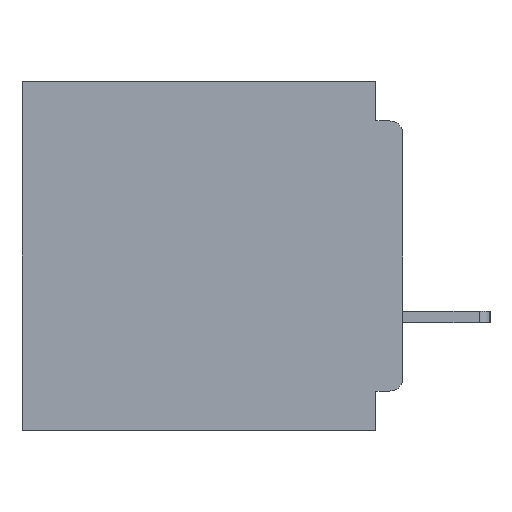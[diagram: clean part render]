
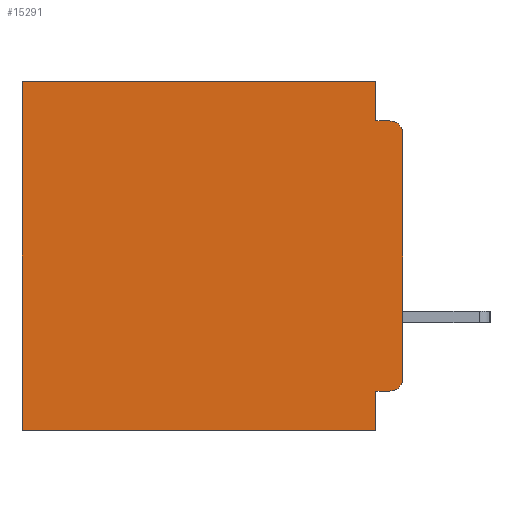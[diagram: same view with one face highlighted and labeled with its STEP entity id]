
A CAD part, left-side view. The second image highlights one B-rep face of the part: STEP entity #15291.
In plain terms, the highlighted planar face has unit normal (-1, 0, 0).
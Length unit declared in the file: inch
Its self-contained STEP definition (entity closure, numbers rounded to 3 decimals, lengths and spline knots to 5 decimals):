
#118 = VERTEX_POINT ( 'NONE', #8648 ) ;
#592 = CARTESIAN_POINT ( 'NONE',  ( 0.3, 0.015, -0.34 ) ) ;
#712 = LINE ( 'NONE', #7384, #21413 ) ;
#1091 = DIRECTION ( 'NONE',  ( 0., -1., 0. ) ) ;
#1253 = EDGE_CURVE ( 'NONE', #20576, #32016, #34575, .T. ) ;
#2187 = EDGE_CURVE ( 'NONE', #118, #33348, #6329, .T. ) ;
#2341 = LINE ( 'NONE', #9358, #29979 ) ;
#2576 = ORIENTED_EDGE ( 'NONE', *, *, #2187, .F. ) ;
#2842 = ORIENTED_EDGE ( 'NONE', *, *, #1253, .F. ) ;
#3294 = ORIENTED_EDGE ( 'NONE', *, *, #25798, .T. ) ;
#3337 = ORIENTED_EDGE ( 'NONE', *, *, #29165, .F. ) ;
#3366 = DIRECTION ( 'NONE',  ( 0., 0., -1. ) ) ;
#4216 = CARTESIAN_POINT ( 'NONE',  ( 0.3, 0., -0.34 ) ) ;
#4332 = CARTESIAN_POINT ( 'NONE',  ( 0.3, 0., -0.4 ) ) ;
#4513 = CARTESIAN_POINT ( 'NONE',  ( 0.3, 0.437, -0.4 ) ) ;
#4587 = VERTEX_POINT ( 'NONE', #31724 ) ;
#4635 = CARTESIAN_POINT ( 'NONE',  ( 0.3, 0.031, -0.4 ) ) ;
#5099 = LINE ( 'NONE', #10769, #32546 ) ;
#5153 = ORIENTED_EDGE ( 'NONE', *, *, #20494, .F. ) ;
#5344 = CARTESIAN_POINT ( 'NONE',  ( 0.3, 0., -0.355 ) ) ;
#5604 = DIRECTION ( 'NONE',  ( -1., 0., 0. ) ) ;
#6329 = LINE ( 'NONE', #8721, #26789 ) ;
#6589 = LINE ( 'NONE', #4332, #33174 ) ;
#7053 = DIRECTION ( 'NONE',  ( 0., 1., 0. ) ) ;
#7383 = CARTESIAN_POINT ( 'NONE',  ( 0.3, 0., -0.4 ) ) ;
#7384 = CARTESIAN_POINT ( 'NONE',  ( 0.3, 0.031, 0. ) ) ;
#7402 = EDGE_CURVE ( 'NONE', #33550, #20576, #712, .T. ) ;
#8648 = CARTESIAN_POINT ( 'NONE',  ( 0.3, 0.031, -0.355 ) ) ;
#8721 = CARTESIAN_POINT ( 'NONE',  ( 0.3, 0.031, -0.4 ) ) ;
#9358 = CARTESIAN_POINT ( 'NONE',  ( 0.3, 0.437, -0.4 ) ) ;
#9608 = CIRCLE ( 'NONE', #10340, 0.015 ) ;
#9758 = VECTOR ( 'NONE', #10749, 39.37008 ) ;
#10077 = DIRECTION ( 'NONE',  ( 0., 0., -1. ) ) ;
#10340 = AXIS2_PLACEMENT_3D ( 'NONE', #21699, #5604, #24357 ) ;
#10695 = EDGE_CURVE ( 'NONE', #22828, #118, #16925, .T. ) ;
#10749 = DIRECTION ( 'NONE',  ( 0., 1., 0. ) ) ;
#10769 = CARTESIAN_POINT ( 'NONE',  ( 0.3, 0., -0.4 ) ) ;
#12237 = VERTEX_POINT ( 'NONE', #4513 ) ;
#12695 = ORIENTED_EDGE ( 'NONE', *, *, #17562, .T. ) ;
#12764 = VERTEX_POINT ( 'NONE', #4216 ) ;
#14082 = CARTESIAN_POINT ( 'NONE',  ( 0.3, 0., -0.045 ) ) ;
#15047 = CARTESIAN_POINT ( 'NONE',  ( 0.3, 0., 0. ) ) ;
#15287 = AXIS2_PLACEMENT_3D ( 'NONE', #592, #19508, #3366 ) ;
#15291 = ADVANCED_FACE ( 'NONE', ( #20245 ), #18081, .F. ) ;
#15831 = ORIENTED_EDGE ( 'NONE', *, *, #25248, .T. ) ;
#16299 = CARTESIAN_POINT ( 'NONE',  ( 0.3, 0.031, 0. ) ) ;
#16925 = LINE ( 'NONE', #5344, #9758 ) ;
#17021 = AXIS2_PLACEMENT_3D ( 'NONE', #7383, #26078, #10077 ) ;
#17562 = EDGE_CURVE ( 'NONE', #24877, #12237, #2341, .T. ) ;
#17748 = ORIENTED_EDGE ( 'NONE', *, *, #28412, .T. ) ;
#18081 = PLANE ( 'NONE',  #17021 ) ;
#18260 = ORIENTED_EDGE ( 'NONE', *, *, #10695, .F. ) ;
#19508 = DIRECTION ( 'NONE',  ( -1., 0., 0. ) ) ;
#20160 = DIRECTION ( 'NONE',  ( 0., 0., -1. ) ) ;
#20245 = FACE_OUTER_BOUND ( 'NONE', #34490, .T. ) ;
#20459 = CARTESIAN_POINT ( 'NONE',  ( 0.3, 0.437, 0. ) ) ;
#20494 = EDGE_CURVE ( 'NONE', #33348, #12237, #6589, .T. ) ;
#20576 = VERTEX_POINT ( 'NONE', #31248 ) ;
#20683 = VECTOR ( 'NONE', #1091, 39.37008 ) ;
#21413 = VECTOR ( 'NONE', #24795, 39.37008 ) ;
#21699 = CARTESIAN_POINT ( 'NONE',  ( 0.3, 0.015, -0.06 ) ) ;
#22828 = VERTEX_POINT ( 'NONE', #28586 ) ;
#23194 = ORIENTED_EDGE ( 'NONE', *, *, #7402, .F. ) ;
#24061 = LINE ( 'NONE', #15047, #31017 ) ;
#24184 = DIRECTION ( 'NONE',  ( 0., 0., -1. ) ) ;
#24357 = DIRECTION ( 'NONE',  ( 0., 0., -1. ) ) ;
#24795 = DIRECTION ( 'NONE',  ( 0., 0., -1. ) ) ;
#24877 = VERTEX_POINT ( 'NONE', #20459 ) ;
#25248 = EDGE_CURVE ( 'NONE', #22828, #12764, #27162, .T. ) ;
#25798 = EDGE_CURVE ( 'NONE', #4587, #32016, #9608, .T. ) ;
#26078 = DIRECTION ( 'NONE',  ( 1., 0., 0. ) ) ;
#26735 = DIRECTION ( 'NONE',  ( 0., 0., -1. ) ) ;
#26789 = VECTOR ( 'NONE', #24184, 39.37008 ) ;
#27162 = CIRCLE ( 'NONE', #15287, 0.015 ) ;
#28412 = EDGE_CURVE ( 'NONE', #33550, #24877, #24061, .T. ) ;
#28586 = CARTESIAN_POINT ( 'NONE',  ( 0.3, 0.015, -0.355 ) ) ;
#29165 = EDGE_CURVE ( 'NONE', #4587, #12764, #5099, .T. ) ;
#29979 = VECTOR ( 'NONE', #20160, 39.37008 ) ;
#30841 = CARTESIAN_POINT ( 'NONE',  ( 0.3, 0.015, -0.045 ) ) ;
#31017 = VECTOR ( 'NONE', #33499, 39.37008 ) ;
#31248 = CARTESIAN_POINT ( 'NONE',  ( 0.3, 0.031, -0.045 ) ) ;
#31724 = CARTESIAN_POINT ( 'NONE',  ( 0.3, 0., -0.06 ) ) ;
#32016 = VERTEX_POINT ( 'NONE', #30841 ) ;
#32546 = VECTOR ( 'NONE', #26735, 39.37008 ) ;
#33174 = VECTOR ( 'NONE', #7053, 39.37008 ) ;
#33348 = VERTEX_POINT ( 'NONE', #4635 ) ;
#33499 = DIRECTION ( 'NONE',  ( 0., 1., 0. ) ) ;
#33550 = VERTEX_POINT ( 'NONE', #16299 ) ;
#34490 = EDGE_LOOP ( 'NONE', ( #3337, #3294, #2842, #23194, #17748, #12695, #5153, #2576, #18260, #15831 ) ) ;
#34575 = LINE ( 'NONE', #14082, #20683 ) ;
